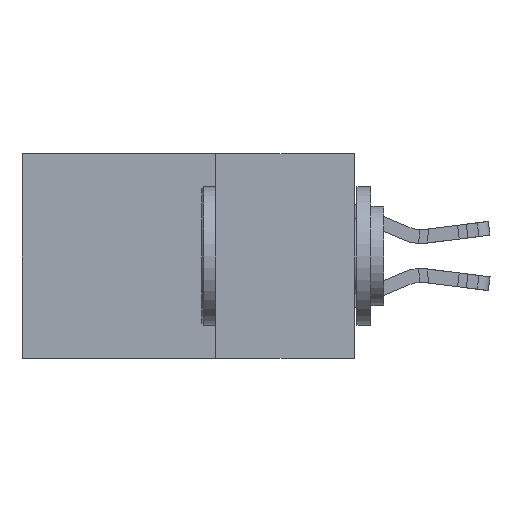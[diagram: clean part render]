
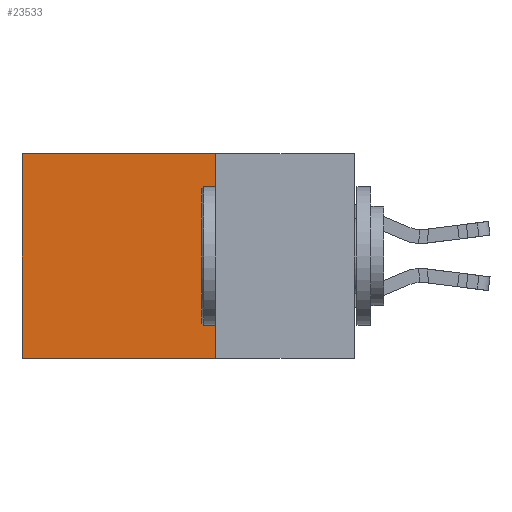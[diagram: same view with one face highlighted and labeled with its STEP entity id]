
A CAD part, left-side view. The second image highlights one B-rep face of the part: STEP entity #23533.
In plain terms, the highlighted planar face has unit normal (-1, 0, 0).
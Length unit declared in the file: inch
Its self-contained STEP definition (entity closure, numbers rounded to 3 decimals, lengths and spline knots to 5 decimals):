
#607 = CARTESIAN_POINT ( 'NONE',  ( 0.2615, 0.25, -0.37 ) ) ;
#857 = EDGE_CURVE ( 'NONE', #7069, #3981, #7715, .T. ) ;
#1672 = DIRECTION ( 'NONE',  ( 0., 1., 0. ) ) ;
#2809 = CARTESIAN_POINT ( 'NONE',  ( 0.2615, 0.6, -0.37 ) ) ;
#2958 = AXIS2_PLACEMENT_3D ( 'NONE', #24674, #12249, #26747 ) ;
#3758 = VERTEX_POINT ( 'NONE', #11634 ) ;
#3981 = VERTEX_POINT ( 'NONE', #2809 ) ;
#4993 = LINE ( 'NONE', #607, #15394 ) ;
#5924 = CARTESIAN_POINT ( 'NONE',  ( 0.2615, 0.25, 0. ) ) ;
#6021 = VECTOR ( 'NONE', #1672, 39.37008 ) ;
#7069 = VERTEX_POINT ( 'NONE', #26180 ) ;
#7715 = LINE ( 'NONE', #11535, #24896 ) ;
#7802 = EDGE_CURVE ( 'NONE', #3758, #26451, #22607, .T. ) ;
#8234 = ORIENTED_EDGE ( 'NONE', *, *, #21073, .F. ) ;
#8377 = CARTESIAN_POINT ( 'NONE',  ( 0.2615, 0.6, -0.37 ) ) ;
#11535 = CARTESIAN_POINT ( 'NONE',  ( 0.2615, 0.25, -0.37 ) ) ;
#11634 = CARTESIAN_POINT ( 'NONE',  ( 0.2615, 0.25, 0. ) ) ;
#12166 = PLANE ( 'NONE',  #2958 ) ;
#12249 = DIRECTION ( 'NONE',  ( 1., 0., 0. ) ) ;
#12510 = EDGE_CURVE ( 'NONE', #26451, #3981, #19069, .T. ) ;
#12973 = CARTESIAN_POINT ( 'NONE',  ( 0.2615, 0.6, 0. ) ) ;
#13539 = VECTOR ( 'NONE', #24405, 39.37008 ) ;
#14636 = EDGE_LOOP ( 'NONE', ( #15084, #20885, #8234, #15596 ) ) ;
#15084 = ORIENTED_EDGE ( 'NONE', *, *, #12510, .T. ) ;
#15343 = DIRECTION ( 'NONE',  ( 0., 0., -1. ) ) ;
#15394 = VECTOR ( 'NONE', #15343, 39.37008 ) ;
#15596 = ORIENTED_EDGE ( 'NONE', *, *, #7802, .T. ) ;
#15608 = FACE_OUTER_BOUND ( 'NONE', #14636, .T. ) ;
#18674 = DIRECTION ( 'NONE',  ( 0., 1., 0. ) ) ;
#19069 = LINE ( 'NONE', #8377, #13539 ) ;
#20885 = ORIENTED_EDGE ( 'NONE', *, *, #857, .F. ) ;
#21073 = EDGE_CURVE ( 'NONE', #3758, #7069, #4993, .T. ) ;
#22607 = LINE ( 'NONE', #5924, #6021 ) ;
#23533 = ADVANCED_FACE ( 'NONE', ( #15608 ), #12166, .F. ) ;
#24405 = DIRECTION ( 'NONE',  ( 0., 0., -1. ) ) ;
#24674 = CARTESIAN_POINT ( 'NONE',  ( 0.2615, 0.25, -0.37 ) ) ;
#24896 = VECTOR ( 'NONE', #18674, 39.37008 ) ;
#26180 = CARTESIAN_POINT ( 'NONE',  ( 0.2615, 0.25, -0.37 ) ) ;
#26451 = VERTEX_POINT ( 'NONE', #12973 ) ;
#26747 = DIRECTION ( 'NONE',  ( 0., 0., -1. ) ) ;
